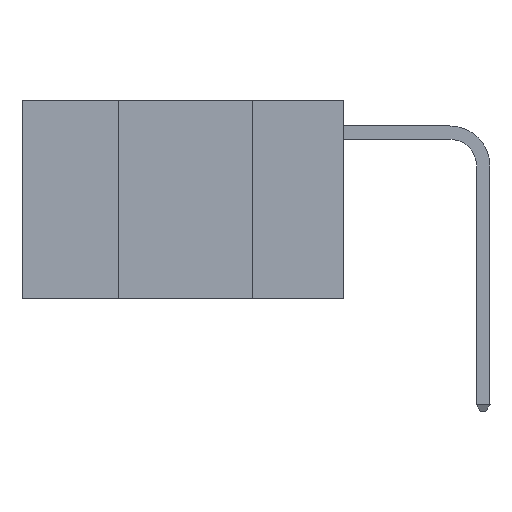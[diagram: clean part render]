
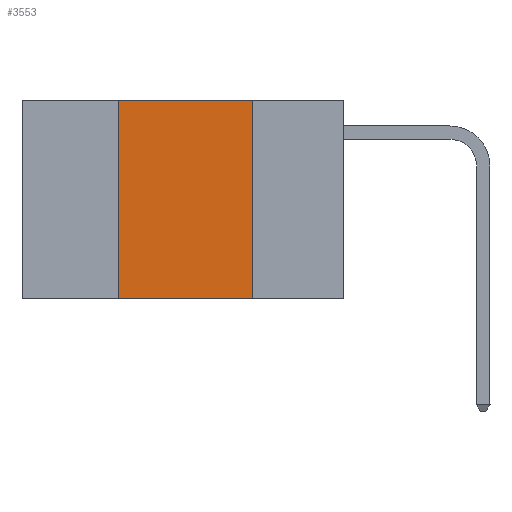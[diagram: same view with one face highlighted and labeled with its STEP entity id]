
A CAD part, left-side view. The second image highlights one B-rep face of the part: STEP entity #3553.
In plain terms, the highlighted planar face has unit normal (-1, 0, 0).
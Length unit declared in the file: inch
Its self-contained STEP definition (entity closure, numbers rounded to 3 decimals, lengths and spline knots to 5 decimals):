
#93 = VECTOR ( 'NONE', #15882, 39.37008 ) ;
#132 = LINE ( 'NONE', #2593, #16042 ) ;
#190 = DIRECTION ( 'NONE',  ( 0., 0., -1. ) ) ;
#497 = LINE ( 'NONE', #8396, #93 ) ;
#861 = CARTESIAN_POINT ( 'NONE',  ( 0., 0.42, 0. ) ) ;
#1822 = ORIENTED_EDGE ( 'NONE', *, *, #7373, .F. ) ;
#2066 = CARTESIAN_POINT ( 'NONE',  ( 0., 0.17, -0.37 ) ) ;
#2593 = CARTESIAN_POINT ( 'NONE',  ( 0., 0.6, -0.37 ) ) ;
#3520 = AXIS2_PLACEMENT_3D ( 'NONE', #8943, #7742, #190 ) ;
#3553 = ADVANCED_FACE ( 'NONE', ( #5132 ), #6450, .F. ) ;
#3742 = VERTEX_POINT ( 'NONE', #11873 ) ;
#3850 = DIRECTION ( 'NONE',  ( 0., -1., 0. ) ) ;
#4511 = VERTEX_POINT ( 'NONE', #2066 ) ;
#5132 = FACE_OUTER_BOUND ( 'NONE', #15353, .T. ) ;
#6450 = PLANE ( 'NONE',  #3520 ) ;
#6744 = CARTESIAN_POINT ( 'NONE',  ( 0., 0.17, 0. ) ) ;
#6779 = LINE ( 'NONE', #861, #10146 ) ;
#7123 = CARTESIAN_POINT ( 'NONE',  ( 0., 0.42, 0. ) ) ;
#7357 = EDGE_CURVE ( 'NONE', #3742, #10621, #6779, .T. ) ;
#7373 = EDGE_CURVE ( 'NONE', #10621, #12268, #497, .T. ) ;
#7742 = DIRECTION ( 'NONE',  ( 1., 0., 0. ) ) ;
#8095 = ORIENTED_EDGE ( 'NONE', *, *, #14782, .F. ) ;
#8396 = CARTESIAN_POINT ( 'NONE',  ( 0., 0.6, 0. ) ) ;
#8934 = LINE ( 'NONE', #6744, #11855 ) ;
#8943 = CARTESIAN_POINT ( 'NONE',  ( 0., 0.6, 0. ) ) ;
#9279 = ORIENTED_EDGE ( 'NONE', *, *, #13183, .T. ) ;
#9652 = DIRECTION ( 'NONE',  ( 0., 0., 1. ) ) ;
#10146 = VECTOR ( 'NONE', #9652, 39.37008 ) ;
#10621 = VERTEX_POINT ( 'NONE', #7123 ) ;
#11855 = VECTOR ( 'NONE', #13062, 39.37008 ) ;
#11873 = CARTESIAN_POINT ( 'NONE',  ( 0., 0.42, -0.37 ) ) ;
#12200 = ORIENTED_EDGE ( 'NONE', *, *, #7357, .F. ) ;
#12268 = VERTEX_POINT ( 'NONE', #15764 ) ;
#13062 = DIRECTION ( 'NONE',  ( 0., 0., -1. ) ) ;
#13183 = EDGE_CURVE ( 'NONE', #3742, #4511, #132, .T. ) ;
#14782 = EDGE_CURVE ( 'NONE', #12268, #4511, #8934, .T. ) ;
#15353 = EDGE_LOOP ( 'NONE', ( #8095, #1822, #12200, #9279 ) ) ;
#15764 = CARTESIAN_POINT ( 'NONE',  ( 0., 0.17, 0. ) ) ;
#15882 = DIRECTION ( 'NONE',  ( 0., -1., 0. ) ) ;
#16042 = VECTOR ( 'NONE', #3850, 39.37008 ) ;
